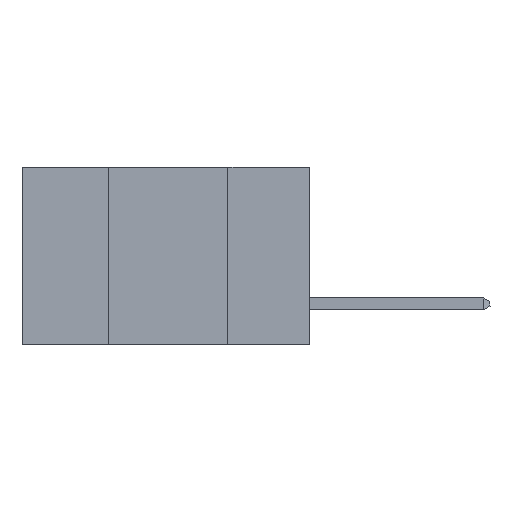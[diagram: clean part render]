
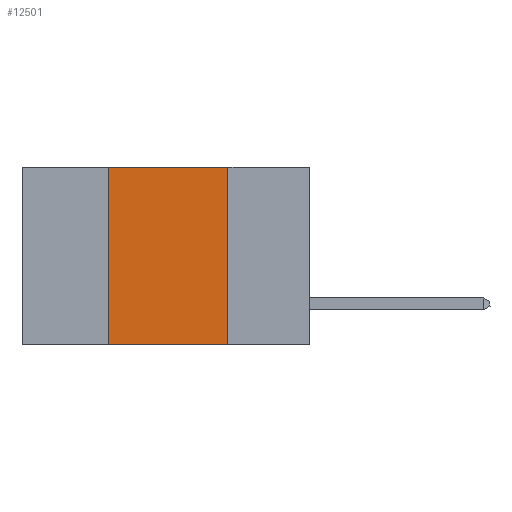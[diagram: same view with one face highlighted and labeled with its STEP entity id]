
A CAD part, left-side view. The second image highlights one B-rep face of the part: STEP entity #12501.
In plain terms, the highlighted planar face has unit normal (-1, 0, 0).
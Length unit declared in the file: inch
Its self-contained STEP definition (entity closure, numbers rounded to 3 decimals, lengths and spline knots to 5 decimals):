
#199 = EDGE_CURVE ( 'NONE', #24624, #13687, #14020, .T. ) ;
#853 = EDGE_CURVE ( 'NONE', #15276, #7463, #17241, .T. ) ;
#1576 = CARTESIAN_POINT ( 'NONE',  ( 0., 0.42, 0. ) ) ;
#2470 = CARTESIAN_POINT ( 'NONE',  ( 0., 0.17, -0.37 ) ) ;
#2886 = ORIENTED_EDGE ( 'NONE', *, *, #199, .F. ) ;
#3160 = CARTESIAN_POINT ( 'NONE',  ( 0., 0.42, 0. ) ) ;
#4471 = FACE_OUTER_BOUND ( 'NONE', #20866, .T. ) ;
#4477 = AXIS2_PLACEMENT_3D ( 'NONE', #24553, #12233, #26624 ) ;
#5215 = CARTESIAN_POINT ( 'NONE',  ( 0., 0.6, -0.37 ) ) ;
#5225 = CARTESIAN_POINT ( 'NONE',  ( 0., 0.42, -0.37 ) ) ;
#5231 = LINE ( 'NONE', #19848, #20487 ) ;
#5250 = DIRECTION ( 'NONE',  ( 0., -1., 0. ) ) ;
#6474 = EDGE_CURVE ( 'NONE', #15276, #24624, #19687, .T. ) ;
#7463 = VERTEX_POINT ( 'NONE', #2470 ) ;
#7504 = DIRECTION ( 'NONE',  ( 0., 0., -1. ) ) ;
#8817 = ORIENTED_EDGE ( 'NONE', *, *, #9692, .F. ) ;
#9303 = VECTOR ( 'NONE', #15714, 39.37008 ) ;
#9347 = CARTESIAN_POINT ( 'NONE',  ( 0., 0.6, 0. ) ) ;
#9692 = EDGE_CURVE ( 'NONE', #13687, #7463, #5231, .T. ) ;
#12233 = DIRECTION ( 'NONE',  ( 1., 0., 0. ) ) ;
#12501 = ADVANCED_FACE ( 'NONE', ( #4471 ), #20448, .F. ) ;
#13687 = VERTEX_POINT ( 'NONE', #13804 ) ;
#13767 = ORIENTED_EDGE ( 'NONE', *, *, #6474, .F. ) ;
#13804 = CARTESIAN_POINT ( 'NONE',  ( 0., 0.17, 0. ) ) ;
#14020 = LINE ( 'NONE', #9347, #18858 ) ;
#15276 = VERTEX_POINT ( 'NONE', #5225 ) ;
#15714 = DIRECTION ( 'NONE',  ( 0., 0., 1. ) ) ;
#16621 = ORIENTED_EDGE ( 'NONE', *, *, #853, .T. ) ;
#17241 = LINE ( 'NONE', #5215, #22033 ) ;
#17698 = DIRECTION ( 'NONE',  ( 0., -1., 0. ) ) ;
#18858 = VECTOR ( 'NONE', #5250, 39.37008 ) ;
#19687 = LINE ( 'NONE', #3160, #9303 ) ;
#19848 = CARTESIAN_POINT ( 'NONE',  ( 0., 0.17, 0. ) ) ;
#20448 = PLANE ( 'NONE',  #4477 ) ;
#20487 = VECTOR ( 'NONE', #7504, 39.37008 ) ;
#20866 = EDGE_LOOP ( 'NONE', ( #8817, #2886, #13767, #16621 ) ) ;
#22033 = VECTOR ( 'NONE', #17698, 39.37008 ) ;
#24553 = CARTESIAN_POINT ( 'NONE',  ( 0., 0.6, 0. ) ) ;
#24624 = VERTEX_POINT ( 'NONE', #1576 ) ;
#26624 = DIRECTION ( 'NONE',  ( 0., 0., -1. ) ) ;
